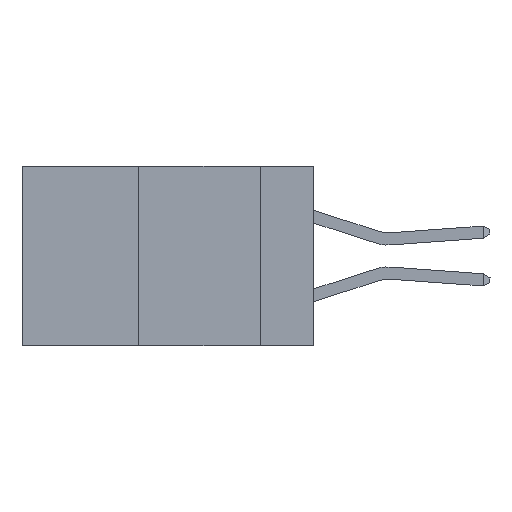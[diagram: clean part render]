
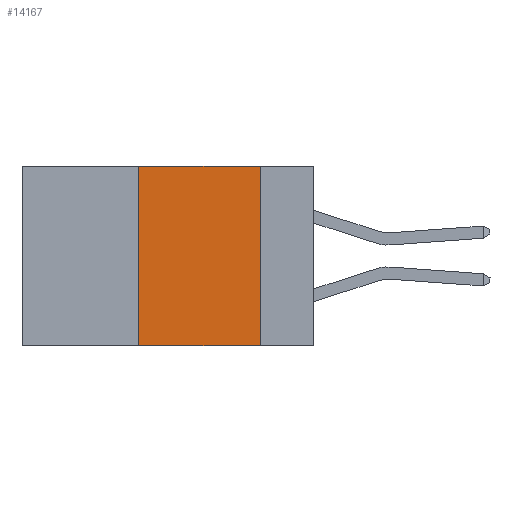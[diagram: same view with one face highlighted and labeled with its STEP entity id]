
A CAD part, left-side view. The second image highlights one B-rep face of the part: STEP entity #14167.
In plain terms, the highlighted planar face has unit normal (-1, 0, 0).
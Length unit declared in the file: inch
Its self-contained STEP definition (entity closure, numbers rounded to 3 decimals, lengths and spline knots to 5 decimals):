
#92 = EDGE_LOOP ( 'NONE', ( #191, #245, #451, #500 ) ) ;
#157 = AXIS2_PLACEMENT_3D ( 'NONE', #6429, #14667, #7628 ) ;
#191 = ORIENTED_EDGE ( 'NONE', *, *, #5859, .F. ) ;
#245 = ORIENTED_EDGE ( 'NONE', *, *, #4146, .F. ) ;
#451 = ORIENTED_EDGE ( 'NONE', *, *, #2540, .F. ) ;
#500 = ORIENTED_EDGE ( 'NONE', *, *, #11267, .T. ) ;
#982 = VECTOR ( 'NONE', #8182, 39.37008 ) ;
#1269 = CARTESIAN_POINT ( 'NONE',  ( 0., 0.11, -0.37 ) ) ;
#1949 = VERTEX_POINT ( 'NONE', #9526 ) ;
#2298 = VERTEX_POINT ( 'NONE', #1269 ) ;
#2540 = EDGE_CURVE ( 'NONE', #11562, #15517, #14495, .T. ) ;
#2574 = CARTESIAN_POINT ( 'NONE',  ( 0., 0.36, 0. ) ) ;
#3135 = DIRECTION ( 'NONE',  ( 0., 0., 1. ) ) ;
#4146 = EDGE_CURVE ( 'NONE', #15517, #1949, #8587, .T. ) ;
#5045 = VECTOR ( 'NONE', #3135, 39.37008 ) ;
#5859 = EDGE_CURVE ( 'NONE', #1949, #2298, #13497, .T. ) ;
#6429 = CARTESIAN_POINT ( 'NONE',  ( 0., 0.6, 0. ) ) ;
#6972 = CARTESIAN_POINT ( 'NONE',  ( 0., 0.36, 0. ) ) ;
#7435 = CARTESIAN_POINT ( 'NONE',  ( 0., 0.36, -0.37 ) ) ;
#7628 = DIRECTION ( 'NONE',  ( 0., 0., -1. ) ) ;
#8182 = DIRECTION ( 'NONE',  ( 0., -1., 0. ) ) ;
#8587 = LINE ( 'NONE', #9254, #11771 ) ;
#9254 = CARTESIAN_POINT ( 'NONE',  ( 0., 0.6, 0. ) ) ;
#9404 = DIRECTION ( 'NONE',  ( 0., -1., 0. ) ) ;
#9526 = CARTESIAN_POINT ( 'NONE',  ( 0., 0.11, 0. ) ) ;
#9989 = PLANE ( 'NONE',  #157 ) ;
#10399 = VECTOR ( 'NONE', #12830, 39.37008 ) ;
#11267 = EDGE_CURVE ( 'NONE', #11562, #2298, #13871, .T. ) ;
#11562 = VERTEX_POINT ( 'NONE', #7435 ) ;
#11771 = VECTOR ( 'NONE', #9404, 39.37008 ) ;
#12830 = DIRECTION ( 'NONE',  ( 0., 0., -1. ) ) ;
#13075 = CARTESIAN_POINT ( 'NONE',  ( 0., 0.11, 0. ) ) ;
#13497 = LINE ( 'NONE', #13075, #10399 ) ;
#13871 = LINE ( 'NONE', #14040, #982 ) ;
#14040 = CARTESIAN_POINT ( 'NONE',  ( 0., 0.6, -0.37 ) ) ;
#14167 = ADVANCED_FACE ( 'NONE', ( #15179 ), #9989, .F. ) ;
#14495 = LINE ( 'NONE', #2574, #5045 ) ;
#14667 = DIRECTION ( 'NONE',  ( 1., 0., 0. ) ) ;
#15179 = FACE_OUTER_BOUND ( 'NONE', #92, .T. ) ;
#15517 = VERTEX_POINT ( 'NONE', #6972 ) ;
